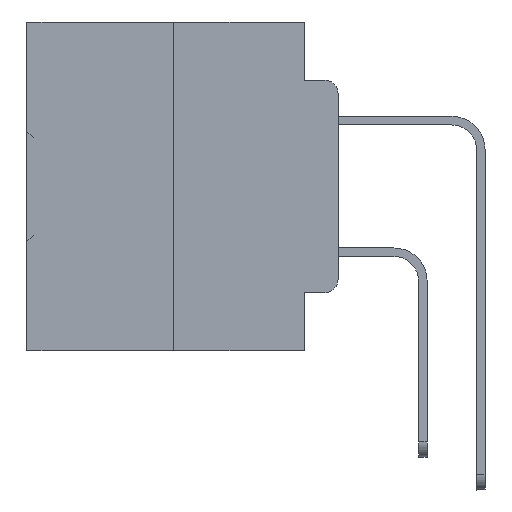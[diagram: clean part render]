
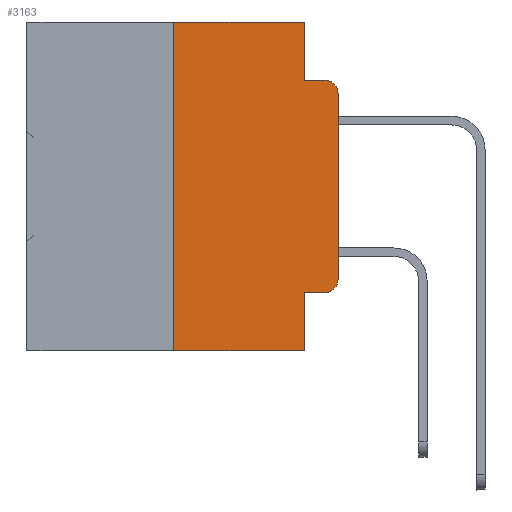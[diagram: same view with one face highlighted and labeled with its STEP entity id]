
A CAD part, left-side view. The second image highlights one B-rep face of the part: STEP entity #3163.
In plain terms, the highlighted planar face has unit normal (-1, 0, 0).
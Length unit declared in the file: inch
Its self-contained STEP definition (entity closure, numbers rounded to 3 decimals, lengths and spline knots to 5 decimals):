
#437 = DIRECTION ( 'NONE',  ( 0., -1., 0. ) ) ;
#856 = VECTOR ( 'NONE', #15943, 39.37008 ) ;
#914 = CARTESIAN_POINT ( 'NONE',  ( 0., 0.25, 0. ) ) ;
#957 = ORIENTED_EDGE ( 'NONE', *, *, #21224, .F. ) ;
#1533 = VERTEX_POINT ( 'NONE', #39082 ) ;
#3027 = VECTOR ( 'NONE', #17547, 39.37008 ) ;
#3083 = CARTESIAN_POINT ( 'NONE',  ( 0., 0.25, -0.5 ) ) ;
#3163 = ADVANCED_FACE ( 'NONE', ( #37563 ), #28935, .F. ) ;
#3681 = CARTESIAN_POINT ( 'NONE',  ( 0., 0.02, -0.4115 ) ) ;
#3838 = LINE ( 'NONE', #20579, #35062 ) ;
#3923 = EDGE_CURVE ( 'NONE', #15428, #7398, #11172, .T. ) ;
#4140 = VECTOR ( 'NONE', #28225, 39.37008 ) ;
#6354 = LINE ( 'NONE', #18975, #29667 ) ;
#6562 = CARTESIAN_POINT ( 'NONE',  ( 0., 0.051, -0.0885 ) ) ;
#6592 = DIRECTION ( 'NONE',  ( 0., 0., -1. ) ) ;
#7025 = VERTEX_POINT ( 'NONE', #3681 ) ;
#7398 = VERTEX_POINT ( 'NONE', #36037 ) ;
#8010 = CARTESIAN_POINT ( 'NONE',  ( 0., 0.051, -0.5 ) ) ;
#8533 = EDGE_CURVE ( 'NONE', #14893, #13647, #3838, .T. ) ;
#8850 = CARTESIAN_POINT ( 'NONE',  ( 0., 0.051, -0.4115 ) ) ;
#9120 = CARTESIAN_POINT ( 'NONE',  ( 0., 0.051, 0. ) ) ;
#9863 = DIRECTION ( 'NONE',  ( -1., 0., 0. ) ) ;
#10739 = DIRECTION ( 'NONE',  ( 1., 0., 0. ) ) ;
#11172 = LINE ( 'NONE', #35325, #3027 ) ;
#11236 = CARTESIAN_POINT ( 'NONE',  ( 0., 0.051, 0. ) ) ;
#11440 = AXIS2_PLACEMENT_3D ( 'NONE', #28122, #9863, #31083 ) ;
#11445 = VERTEX_POINT ( 'NONE', #11236 ) ;
#12101 = VECTOR ( 'NONE', #27306, 39.37008 ) ;
#12247 = CARTESIAN_POINT ( 'NONE',  ( 0., 0.02, -0.1085 ) ) ;
#12537 = VERTEX_POINT ( 'NONE', #29753 ) ;
#13647 = VERTEX_POINT ( 'NONE', #8010 ) ;
#14720 = ORIENTED_EDGE ( 'NONE', *, *, #19136, .F. ) ;
#14893 = VERTEX_POINT ( 'NONE', #3083 ) ;
#15024 = EDGE_CURVE ( 'NONE', #7025, #15428, #19411, .T. ) ;
#15261 = VECTOR ( 'NONE', #437, 39.37008 ) ;
#15375 = DIRECTION ( 'NONE',  ( 0., 0., -1. ) ) ;
#15428 = VERTEX_POINT ( 'NONE', #20977 ) ;
#15943 = DIRECTION ( 'NONE',  ( 0., -1., 0. ) ) ;
#16724 = ORIENTED_EDGE ( 'NONE', *, *, #33127, .F. ) ;
#17547 = DIRECTION ( 'NONE',  ( 0., 0., 1. ) ) ;
#17702 = ORIENTED_EDGE ( 'NONE', *, *, #31138, .F. ) ;
#18085 = VERTEX_POINT ( 'NONE', #914 ) ;
#18133 = LINE ( 'NONE', #9120, #32989 ) ;
#18331 = CARTESIAN_POINT ( 'NONE',  ( 0., 0.25, 0. ) ) ;
#18975 = CARTESIAN_POINT ( 'NONE',  ( 0., 0.051, 0. ) ) ;
#19136 = EDGE_CURVE ( 'NONE', #18085, #11445, #39046, .T. ) ;
#19236 = EDGE_CURVE ( 'NONE', #23515, #7025, #28451, .T. ) ;
#19411 = CIRCLE ( 'NONE', #11440, 0.02 ) ;
#20012 = CARTESIAN_POINT ( 'NONE',  ( 0., 0.473, 0. ) ) ;
#20579 = CARTESIAN_POINT ( 'NONE',  ( 0., 0.473, -0.5 ) ) ;
#20977 = CARTESIAN_POINT ( 'NONE',  ( 0., 0., -0.3915 ) ) ;
#21224 = EDGE_CURVE ( 'NONE', #23515, #13647, #6354, .T. ) ;
#23515 = VERTEX_POINT ( 'NONE', #8850 ) ;
#24109 = CIRCLE ( 'NONE', #24735, 0.02 ) ;
#24227 = AXIS2_PLACEMENT_3D ( 'NONE', #20012, #10739, #31890 ) ;
#24254 = ORIENTED_EDGE ( 'NONE', *, *, #39022, .T. ) ;
#24536 = DIRECTION ( 'NONE',  ( 0., 0., -1. ) ) ;
#24735 = AXIS2_PLACEMENT_3D ( 'NONE', #12247, #33329, #15375 ) ;
#26245 = LINE ( 'NONE', #6562, #856 ) ;
#27182 = EDGE_CURVE ( 'NONE', #14893, #18085, #27312, .T. ) ;
#27306 = DIRECTION ( 'NONE',  ( 0., 0., 1. ) ) ;
#27312 = LINE ( 'NONE', #18331, #12101 ) ;
#27509 = ORIENTED_EDGE ( 'NONE', *, *, #3923, .T. ) ;
#28122 = CARTESIAN_POINT ( 'NONE',  ( 0., 0.02, -0.3915 ) ) ;
#28225 = DIRECTION ( 'NONE',  ( 0., -1., 0. ) ) ;
#28451 = LINE ( 'NONE', #34182, #4140 ) ;
#28935 = PLANE ( 'NONE',  #24227 ) ;
#29504 = DIRECTION ( 'NONE',  ( 0., -1., 0. ) ) ;
#29667 = VECTOR ( 'NONE', #6592, 39.37008 ) ;
#29753 = CARTESIAN_POINT ( 'NONE',  ( 0., 0.02, -0.0885 ) ) ;
#31083 = DIRECTION ( 'NONE',  ( 0., 0., -1. ) ) ;
#31138 = EDGE_CURVE ( 'NONE', #11445, #1533, #18133, .T. ) ;
#31890 = DIRECTION ( 'NONE',  ( 0., 0., -1. ) ) ;
#32989 = VECTOR ( 'NONE', #24536, 39.37008 ) ;
#33127 = EDGE_CURVE ( 'NONE', #1533, #12537, #26245, .T. ) ;
#33329 = DIRECTION ( 'NONE',  ( -1., 0., 0. ) ) ;
#33799 = CARTESIAN_POINT ( 'NONE',  ( 0., 0.473, 0. ) ) ;
#34182 = CARTESIAN_POINT ( 'NONE',  ( 0., 0.051, -0.4115 ) ) ;
#35062 = VECTOR ( 'NONE', #29504, 39.37008 ) ;
#35269 = ORIENTED_EDGE ( 'NONE', *, *, #8533, .T. ) ;
#35325 = CARTESIAN_POINT ( 'NONE',  ( 0., 0., 0. ) ) ;
#35900 = ORIENTED_EDGE ( 'NONE', *, *, #27182, .F. ) ;
#36037 = CARTESIAN_POINT ( 'NONE',  ( 0., 0., -0.1085 ) ) ;
#36039 = ORIENTED_EDGE ( 'NONE', *, *, #15024, .T. ) ;
#36655 = ORIENTED_EDGE ( 'NONE', *, *, #19236, .T. ) ;
#37563 = FACE_OUTER_BOUND ( 'NONE', #37793, .T. ) ;
#37793 = EDGE_LOOP ( 'NONE', ( #27509, #24254, #16724, #17702, #14720, #35900, #35269, #957, #36655, #36039 ) ) ;
#39022 = EDGE_CURVE ( 'NONE', #7398, #12537, #24109, .T. ) ;
#39046 = LINE ( 'NONE', #33799, #15261 ) ;
#39082 = CARTESIAN_POINT ( 'NONE',  ( 0., 0.051, -0.0885 ) ) ;
